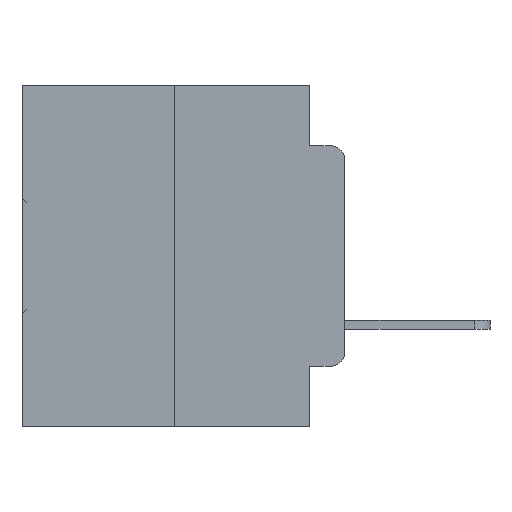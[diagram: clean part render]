
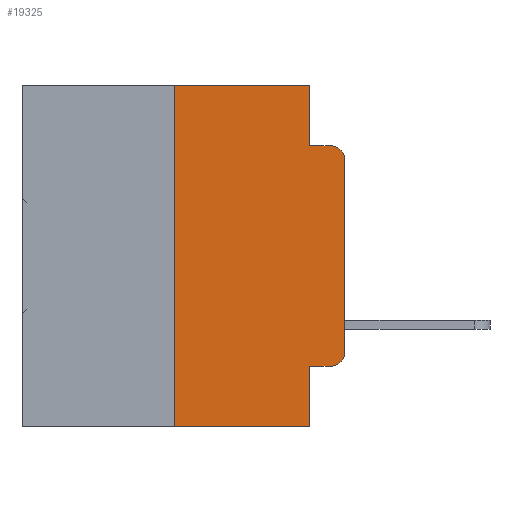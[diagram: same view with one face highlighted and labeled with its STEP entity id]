
A CAD part, left-side view. The second image highlights one B-rep face of the part: STEP entity #19325.
In plain terms, the highlighted planar face has unit normal (-1, 0, 0).
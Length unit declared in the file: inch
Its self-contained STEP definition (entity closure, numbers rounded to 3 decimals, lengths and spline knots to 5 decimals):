
#1098 = LINE ( 'NONE', #32214, #15595 ) ;
#1414 = CARTESIAN_POINT ( 'NONE',  ( 0., 0.051, 0. ) ) ;
#2835 = VERTEX_POINT ( 'NONE', #18986 ) ;
#3387 = EDGE_CURVE ( 'NONE', #29445, #20835, #7034, .T. ) ;
#3745 = LINE ( 'NONE', #24381, #23104 ) ;
#3842 = CIRCLE ( 'NONE', #17001, 0.02 ) ;
#4317 = DIRECTION ( 'NONE',  ( 1., 0., 0. ) ) ;
#4743 = FACE_OUTER_BOUND ( 'NONE', #12042, .T. ) ;
#5118 = EDGE_CURVE ( 'NONE', #18647, #25492, #7617, .T. ) ;
#5276 = CARTESIAN_POINT ( 'NONE',  ( 0., 0.051, -0.0885 ) ) ;
#5391 = DIRECTION ( 'NONE',  ( 0., -1., 0. ) ) ;
#6051 = DIRECTION ( 'NONE',  ( 0., 0., 1. ) ) ;
#6535 = VERTEX_POINT ( 'NONE', #18913 ) ;
#6717 = DIRECTION ( 'NONE',  ( 0., 0., -1. ) ) ;
#6828 = DIRECTION ( 'NONE',  ( 0., -1., 0. ) ) ;
#7034 = LINE ( 'NONE', #12539, #24663 ) ;
#7072 = ORIENTED_EDGE ( 'NONE', *, *, #15353, .T. ) ;
#7428 = DIRECTION ( 'NONE',  ( -1., 0., 0. ) ) ;
#7447 = DIRECTION ( 'NONE',  ( 0., -1., 0. ) ) ;
#7617 = LINE ( 'NONE', #21130, #26724 ) ;
#8314 = ORIENTED_EDGE ( 'NONE', *, *, #5118, .F. ) ;
#8779 = CARTESIAN_POINT ( 'NONE',  ( 0., 0.473, 0. ) ) ;
#9677 = CARTESIAN_POINT ( 'NONE',  ( 0., 0.051, -0.0885 ) ) ;
#10235 = EDGE_CURVE ( 'NONE', #6535, #29362, #11218, .T. ) ;
#10542 = DIRECTION ( 'NONE',  ( -1., 0., 0. ) ) ;
#11218 = LINE ( 'NONE', #1414, #30212 ) ;
#11263 = DIRECTION ( 'NONE',  ( 0., -1., 0. ) ) ;
#11855 = CARTESIAN_POINT ( 'NONE',  ( 0., 0.473, 0. ) ) ;
#12040 = LINE ( 'NONE', #8779, #30990 ) ;
#12042 = EDGE_LOOP ( 'NONE', ( #26202, #7072, #12994, #28499, #20884, #8314, #28128, #23220, #31157, #13023 ) ) ;
#12539 = CARTESIAN_POINT ( 'NONE',  ( 0., 0.051, 0. ) ) ;
#12994 = ORIENTED_EDGE ( 'NONE', *, *, #13629, .F. ) ;
#13023 = ORIENTED_EDGE ( 'NONE', *, *, #22652, .T. ) ;
#13339 = LINE ( 'NONE', #32291, #31457 ) ;
#13629 = EDGE_CURVE ( 'NONE', #29362, #20910, #17075, .T. ) ;
#14449 = VERTEX_POINT ( 'NONE', #26037 ) ;
#15152 = DIRECTION ( 'NONE',  ( 0., 0., 1. ) ) ;
#15353 = EDGE_CURVE ( 'NONE', #21632, #20910, #3842, .T. ) ;
#15595 = VECTOR ( 'NONE', #7447, 39.37008 ) ;
#16492 = CARTESIAN_POINT ( 'NONE',  ( 0., 0.25, -0.5 ) ) ;
#16742 = CARTESIAN_POINT ( 'NONE',  ( 0., 0.25, 0. ) ) ;
#17001 = AXIS2_PLACEMENT_3D ( 'NONE', #22470, #7428, #24940 ) ;
#17018 = PLANE ( 'NONE',  #18159 ) ;
#17075 = LINE ( 'NONE', #5276, #29322 ) ;
#18159 = AXIS2_PLACEMENT_3D ( 'NONE', #11855, #4317, #21986 ) ;
#18647 = VERTEX_POINT ( 'NONE', #16492 ) ;
#18913 = CARTESIAN_POINT ( 'NONE',  ( 0., 0.051, 0. ) ) ;
#18986 = CARTESIAN_POINT ( 'NONE',  ( 0., 0., -0.3915 ) ) ;
#19325 = ADVANCED_FACE ( 'NONE', ( #4743 ), #17018, .F. ) ;
#20765 = CARTESIAN_POINT ( 'NONE',  ( 0., 0.02, -0.0885 ) ) ;
#20835 = VERTEX_POINT ( 'NONE', #30125 ) ;
#20884 = ORIENTED_EDGE ( 'NONE', *, *, #29788, .F. ) ;
#20910 = VERTEX_POINT ( 'NONE', #20765 ) ;
#21130 = CARTESIAN_POINT ( 'NONE',  ( 0., 0.25, 0. ) ) ;
#21632 = VERTEX_POINT ( 'NONE', #28004 ) ;
#21986 = DIRECTION ( 'NONE',  ( 0., 0., -1. ) ) ;
#22470 = CARTESIAN_POINT ( 'NONE',  ( 0., 0.02, -0.1085 ) ) ;
#22550 = DIRECTION ( 'NONE',  ( 0., 0., -1. ) ) ;
#22652 = EDGE_CURVE ( 'NONE', #14449, #2835, #28021, .T. ) ;
#23104 = VECTOR ( 'NONE', #6828, 39.37008 ) ;
#23220 = ORIENTED_EDGE ( 'NONE', *, *, #3387, .F. ) ;
#23708 = EDGE_CURVE ( 'NONE', #2835, #21632, #13339, .T. ) ;
#24381 = CARTESIAN_POINT ( 'NONE',  ( 0., 0.473, -0.5 ) ) ;
#24663 = VECTOR ( 'NONE', #22550, 39.37008 ) ;
#24940 = DIRECTION ( 'NONE',  ( 0., 0., -1. ) ) ;
#25492 = VERTEX_POINT ( 'NONE', #16742 ) ;
#25507 = CARTESIAN_POINT ( 'NONE',  ( 0., 0.02, -0.3915 ) ) ;
#26037 = CARTESIAN_POINT ( 'NONE',  ( 0., 0.02, -0.4115 ) ) ;
#26202 = ORIENTED_EDGE ( 'NONE', *, *, #23708, .T. ) ;
#26724 = VECTOR ( 'NONE', #6051, 39.37008 ) ;
#27407 = CARTESIAN_POINT ( 'NONE',  ( 0., 0.051, -0.4115 ) ) ;
#27913 = DIRECTION ( 'NONE',  ( 0., 0., -1. ) ) ;
#28004 = CARTESIAN_POINT ( 'NONE',  ( 0., 0., -0.1085 ) ) ;
#28021 = CIRCLE ( 'NONE', #30288, 0.02 ) ;
#28128 = ORIENTED_EDGE ( 'NONE', *, *, #28960, .T. ) ;
#28499 = ORIENTED_EDGE ( 'NONE', *, *, #10235, .F. ) ;
#28960 = EDGE_CURVE ( 'NONE', #18647, #20835, #3745, .T. ) ;
#29322 = VECTOR ( 'NONE', #5391, 39.37008 ) ;
#29362 = VERTEX_POINT ( 'NONE', #9677 ) ;
#29445 = VERTEX_POINT ( 'NONE', #27407 ) ;
#29788 = EDGE_CURVE ( 'NONE', #25492, #6535, #12040, .T. ) ;
#30125 = CARTESIAN_POINT ( 'NONE',  ( 0., 0.051, -0.5 ) ) ;
#30212 = VECTOR ( 'NONE', #6717, 39.37008 ) ;
#30288 = AXIS2_PLACEMENT_3D ( 'NONE', #25507, #10542, #27913 ) ;
#30990 = VECTOR ( 'NONE', #11263, 39.37008 ) ;
#31157 = ORIENTED_EDGE ( 'NONE', *, *, #32369, .T. ) ;
#31457 = VECTOR ( 'NONE', #15152, 39.37008 ) ;
#32214 = CARTESIAN_POINT ( 'NONE',  ( 0., 0.051, -0.4115 ) ) ;
#32291 = CARTESIAN_POINT ( 'NONE',  ( 0., 0., 0. ) ) ;
#32369 = EDGE_CURVE ( 'NONE', #29445, #14449, #1098, .T. ) ;
